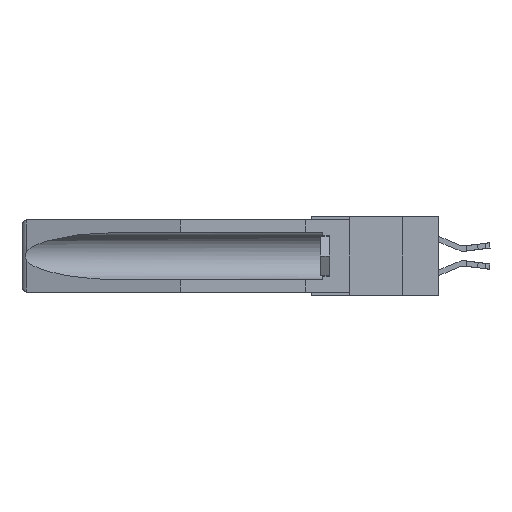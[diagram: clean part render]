
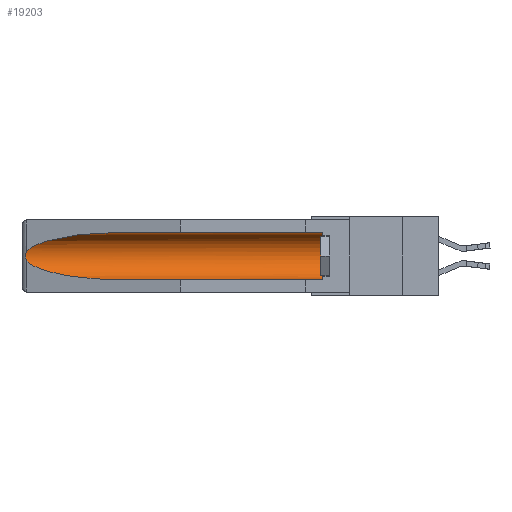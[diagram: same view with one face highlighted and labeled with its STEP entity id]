
A CAD part, left-side view. The second image highlights one B-rep face of the part: STEP entity #19203.
In plain terms, the highlighted cylindrical face has radius 2.857 mm (diameter 5.715 mm), a partial arc.
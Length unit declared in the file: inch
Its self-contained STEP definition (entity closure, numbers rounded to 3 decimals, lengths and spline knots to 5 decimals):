
#269 = DIRECTION ( 'NONE',  ( 0., 0., 1. ) ) ;
#1205 = CARTESIAN_POINT ( 'NONE',  ( 0.155, 0.126, -0.284 ) ) ;
#1631 = CARTESIAN_POINT ( 'NONE',  ( 0.2673, 1.53269, -0.17917 ) ) ;
#1700 = CARTESIAN_POINT ( 'NONE',  ( 0.26597, 1.52961, -0.15275 ) ) ;
#1892 = VERTEX_POINT ( 'NONE', #4294 ) ;
#2172 = VECTOR ( 'NONE', #15633, 39.37008 ) ;
#2304 =( BOUNDED_CURVE ( )  B_SPLINE_CURVE ( 3, ( #10573, #20684, #10857, #13935 ),
 .UNSPECIFIED., .F., .F. ) 
 B_SPLINE_CURVE_WITH_KNOTS ( ( 4, 4 ),
 ( 4.71239, 6.08839 ),
 .UNSPECIFIED. ) 
 CURVE ( )  GEOMETRIC_REPRESENTATION_ITEM ( )  RATIONAL_B_SPLINE_CURVE ( ( 1., 0.848, 0.848, 1. ) ) 
 REPRESENTATION_ITEM ( '' )  );
#3356 = CARTESIAN_POINT ( 'NONE',  ( 0.2673, 1.5327, -0.16383 ) ) ;
#3721 = DIRECTION ( 'NONE',  ( 0., 0., 1. ) ) ;
#4084 = CARTESIAN_POINT ( 'NONE',  ( 0.155, -0.30754, -0.284 ) ) ;
#4178 = CARTESIAN_POINT ( 'NONE',  ( 0.26537, 1.52718, -0.14972 ) ) ;
#4294 = CARTESIAN_POINT ( 'NONE',  ( 0.155, 1.07973, -0.284 ) ) ;
#4468 = EDGE_LOOP ( 'NONE', ( #21127, #4660, #12335, #11434, #7063, #11188 ) ) ;
#4488 = EDGE_CURVE ( 'NONE', #6451, #19095, #20990, .T. ) ;
#4660 = ORIENTED_EDGE ( 'NONE', *, *, #17903, .T. ) ;
#5835 = VERTEX_POINT ( 'NONE', #13082 ) ;
#6451 = VERTEX_POINT ( 'NONE', #18136 ) ;
#6463 = CARTESIAN_POINT ( 'NONE',  ( 0.2675, 1.53308, -0.16763 ) ) ;
#6527 = CIRCLE ( 'NONE', #12980, 0.1125 ) ;
#6542 = CARTESIAN_POINT ( 'NONE',  ( 0.26537, 1.52718, -0.14972 ) ) ;
#6673 = CARTESIAN_POINT ( 'NONE',  ( 0.26597, 1.5296, -0.19026 ) ) ;
#7063 = ORIENTED_EDGE ( 'NONE', *, *, #11435, .T. ) ;
#7321 = B_SPLINE_CURVE_WITH_KNOTS ( 'NONE', 3,
 ( #6542, #1700, #14983, #3356, #6463, #18005, #1631, #14831, #6673, #18145 ),
 .UNSPECIFIED., .F., .F.,
 ( 4, 2, 2, 2, 4 ),
 ( 0., 0.00029, 0.00058, 0.00087, 0.00117 ),
 .UNSPECIFIED. ) ;
#7599 = CARTESIAN_POINT ( 'NONE',  ( 0.21114, 1.30732, -0.284 ) ) ;
#7671 = CARTESIAN_POINT ( 'NONE',  ( 0.25451, 1.48313, -0.24835 ) ) ;
#7913 = VECTOR ( 'NONE', #18302, 39.37008 ) ;
#9058 = FACE_OUTER_BOUND ( 'NONE', #4468, .T. ) ;
#10573 = CARTESIAN_POINT ( 'NONE',  ( 0.155, 1.07973, -0.059 ) ) ;
#10857 = CARTESIAN_POINT ( 'NONE',  ( 0.25451, 1.48313, -0.09465 ) ) ;
#10871 = CARTESIAN_POINT ( 'NONE',  ( 0.155, 1.07973, -0.284 ) ) ;
#11188 = ORIENTED_EDGE ( 'NONE', *, *, #4488, .T. ) ;
#11434 = ORIENTED_EDGE ( 'NONE', *, *, #13723, .F. ) ;
#11435 = EDGE_CURVE ( 'NONE', #12390, #6451, #6527, .T. ) ;
#11773 = DIRECTION ( 'NONE',  ( 0., 1., 0. ) ) ;
#12335 = ORIENTED_EDGE ( 'NONE', *, *, #14615, .T. ) ;
#12390 = VERTEX_POINT ( 'NONE', #1205 ) ;
#12980 = AXIS2_PLACEMENT_3D ( 'NONE', #13525, #19927, #3721 ) ;
#13082 = CARTESIAN_POINT ( 'NONE',  ( 0.26537, 1.52718, -0.19328 ) ) ;
#13472 = CARTESIAN_POINT ( 'NONE',  ( 0.155, -0.30754, -0.1715 ) ) ;
#13525 = CARTESIAN_POINT ( 'NONE',  ( 0.155, 0.126, -0.1715 ) ) ;
#13723 = EDGE_CURVE ( 'NONE', #12390, #1892, #19612, .T. ) ;
#13935 = CARTESIAN_POINT ( 'NONE',  ( 0.26537, 1.52718, -0.14972 ) ) ;
#14615 = EDGE_CURVE ( 'NONE', #5835, #1892, #19381, .T. ) ;
#14831 = CARTESIAN_POINT ( 'NONE',  ( 0.26655, 1.53094, -0.18657 ) ) ;
#14983 = CARTESIAN_POINT ( 'NONE',  ( 0.26654, 1.53092, -0.15636 ) ) ;
#15234 = EDGE_CURVE ( 'NONE', #19095, #16988, #2304, .T. ) ;
#15633 = DIRECTION ( 'NONE',  ( 0., 1., 0. ) ) ;
#15687 = CARTESIAN_POINT ( 'NONE',  ( 0.26537, 1.52718, -0.19328 ) ) ;
#16161 = CARTESIAN_POINT ( 'NONE',  ( 0.155, 1.07973, -0.059 ) ) ;
#16988 = VERTEX_POINT ( 'NONE', #4178 ) ;
#17294 = CYLINDRICAL_SURFACE ( 'NONE', #19959, 0.1125 ) ;
#17903 = EDGE_CURVE ( 'NONE', #16988, #5835, #7321, .T. ) ;
#18005 = CARTESIAN_POINT ( 'NONE',  ( 0.2675, 1.53308, -0.17534 ) ) ;
#18136 = CARTESIAN_POINT ( 'NONE',  ( 0.155, 0.126, -0.059 ) ) ;
#18145 = CARTESIAN_POINT ( 'NONE',  ( 0.26537, 1.52718, -0.19328 ) ) ;
#18302 = DIRECTION ( 'NONE',  ( 0., 1., 0. ) ) ;
#19095 = VERTEX_POINT ( 'NONE', #16161 ) ;
#19203 = ADVANCED_FACE ( 'NONE', ( #9058 ), #17294, .F. ) ;
#19381 =( BOUNDED_CURVE ( )  B_SPLINE_CURVE ( 3, ( #15687, #7671, #7599, #10871 ),
 .UNSPECIFIED., .F., .F. ) 
 B_SPLINE_CURVE_WITH_KNOTS ( ( 4, 4 ),
 ( 0.1948, 1.5708 ),
 .UNSPECIFIED. ) 
 CURVE ( )  GEOMETRIC_REPRESENTATION_ITEM ( )  RATIONAL_B_SPLINE_CURVE ( ( 1., 0.848, 0.848, 1. ) ) 
 REPRESENTATION_ITEM ( '' )  );
#19612 = LINE ( 'NONE', #4084, #2172 ) ;
#19927 = DIRECTION ( 'NONE',  ( 0., -1., 0. ) ) ;
#19942 = CARTESIAN_POINT ( 'NONE',  ( 0.155, -0.30754, -0.059 ) ) ;
#19959 = AXIS2_PLACEMENT_3D ( 'NONE', #13472, #11773, #269 ) ;
#20684 = CARTESIAN_POINT ( 'NONE',  ( 0.21114, 1.30732, -0.059 ) ) ;
#20990 = LINE ( 'NONE', #19942, #7913 ) ;
#21127 = ORIENTED_EDGE ( 'NONE', *, *, #15234, .T. ) ;
